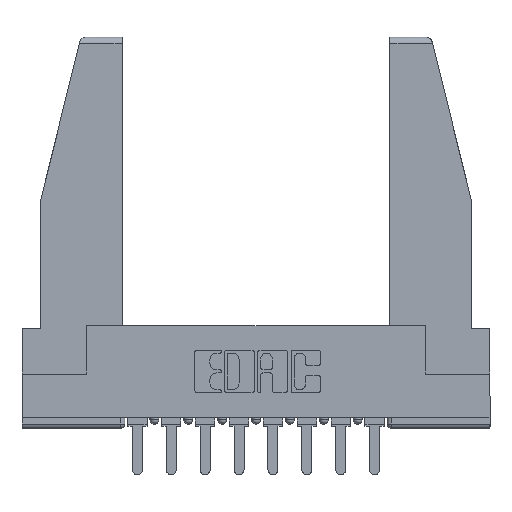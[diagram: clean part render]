
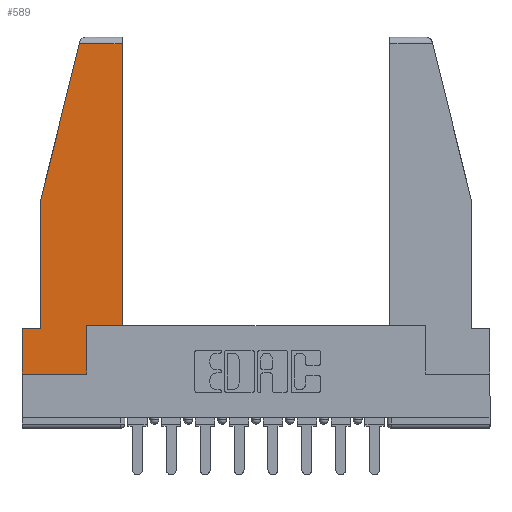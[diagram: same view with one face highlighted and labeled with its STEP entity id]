
A CAD part, top view. The second image highlights one B-rep face of the part: STEP entity #589.
In plain terms, the highlighted planar face has unit normal (0, 0, 1).
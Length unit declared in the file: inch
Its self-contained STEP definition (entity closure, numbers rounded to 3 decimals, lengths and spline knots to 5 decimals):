
#198 = CARTESIAN_POINT ( 'NONE',  ( 0.461, 0.223, 0. ) ) ;
#589 = ADVANCED_FACE ( 'NONE', ( #13682 ), #10594, .T. ) ;
#1011 = DIRECTION ( 'NONE',  ( 0., 1., 0. ) ) ;
#1154 = EDGE_CURVE ( 'NONE', #6235, #12416, #11730, .T. ) ;
#1190 = VERTEX_POINT ( 'NONE', #5610 ) ;
#1563 = LINE ( 'NONE', #4376, #9164 ) ;
#1657 = EDGE_CURVE ( 'NONE', #1190, #8794, #2591, .T. ) ;
#1777 = AXIS2_PLACEMENT_3D ( 'NONE', #8343, #13860, #11594 ) ;
#1882 = EDGE_LOOP ( 'NONE', ( #13280, #6739, #13437, #11659, #7997, #3262, #2547, #11012, #12914 ) ) ;
#1894 = EDGE_CURVE ( 'NONE', #12416, #9973, #11202, .T. ) ;
#2061 = VERTEX_POINT ( 'NONE', #4205 ) ;
#2083 = DIRECTION ( 'NONE',  ( 1., 0., 0. ) ) ;
#2334 = VECTOR ( 'NONE', #7181, 39.37008 ) ;
#2530 = LINE ( 'NONE', #5425, #10459 ) ;
#2544 = EDGE_CURVE ( 'NONE', #8794, #2061, #6162, .T. ) ;
#2547 = ORIENTED_EDGE ( 'NONE', *, *, #13365, .T. ) ;
#2591 = LINE ( 'NONE', #7949, #6899 ) ;
#3027 = LINE ( 'NONE', #4429, #4070 ) ;
#3166 = CARTESIAN_POINT ( 'NONE',  ( 0., 0.21, 0. ) ) ;
#3262 = ORIENTED_EDGE ( 'NONE', *, *, #2544, .T. ) ;
#4070 = VECTOR ( 'NONE', #1011, 39.37008 ) ;
#4136 = VECTOR ( 'NONE', #13581, 39.37008 ) ;
#4205 = CARTESIAN_POINT ( 'NONE',  ( 0., 0., 0. ) ) ;
#4376 = CARTESIAN_POINT ( 'NONE',  ( 0.297, 0.223, 0. ) ) ;
#4429 = CARTESIAN_POINT ( 'NONE',  ( 0.297, 0., 0. ) ) ;
#4791 = VECTOR ( 'NONE', #9503, 39.37008 ) ;
#4915 = LINE ( 'NONE', #12209, #12314 ) ;
#5010 = VECTOR ( 'NONE', #5769, 39.37008 ) ;
#5425 = CARTESIAN_POINT ( 'NONE',  ( 0.271, 1.55, 0. ) ) ;
#5610 = CARTESIAN_POINT ( 'NONE',  ( 0.086, 0.21, 0. ) ) ;
#5612 = CARTESIAN_POINT ( 'NONE',  ( 0.297, 0.223, 0. ) ) ;
#5769 = DIRECTION ( 'NONE',  ( 0., 1., 0. ) ) ;
#6002 = VERTEX_POINT ( 'NONE', #7423 ) ;
#6162 = LINE ( 'NONE', #8306, #4791 ) ;
#6235 = VERTEX_POINT ( 'NONE', #198 ) ;
#6728 = CARTESIAN_POINT ( 'NONE',  ( 0.461, 0.223, 0. ) ) ;
#6739 = ORIENTED_EDGE ( 'NONE', *, *, #1894, .T. ) ;
#6899 = VECTOR ( 'NONE', #13050, 39.37008 ) ;
#7181 = DIRECTION ( 'NONE',  ( 0., -1., 0. ) ) ;
#7215 = CARTESIAN_POINT ( 'NONE',  ( 0.2636, 1.52, 0. ) ) ;
#7249 = EDGE_CURVE ( 'NONE', #11210, #6235, #1563, .T. ) ;
#7423 = CARTESIAN_POINT ( 'NONE',  ( 0.086, 0.8, 0. ) ) ;
#7583 = VERTEX_POINT ( 'NONE', #13689 ) ;
#7949 = CARTESIAN_POINT ( 'NONE',  ( 0., 0.21, 0. ) ) ;
#7997 = ORIENTED_EDGE ( 'NONE', *, *, #1657, .T. ) ;
#8201 = LINE ( 'NONE', #12606, #2334 ) ;
#8306 = CARTESIAN_POINT ( 'NONE',  ( 0., 0.21, 0. ) ) ;
#8343 = CARTESIAN_POINT ( 'NONE',  ( 0., 0., 0. ) ) ;
#8708 = EDGE_CURVE ( 'NONE', #6002, #1190, #8201, .T. ) ;
#8755 = EDGE_CURVE ( 'NONE', #7583, #11210, #3027, .T. ) ;
#8767 = DIRECTION ( 'NONE',  ( 1., 0., 0. ) ) ;
#8794 = VERTEX_POINT ( 'NONE', #3166 ) ;
#9164 = VECTOR ( 'NONE', #2083, 39.37008 ) ;
#9195 = CARTESIAN_POINT ( 'NONE',  ( 0., 1.52, 0. ) ) ;
#9503 = DIRECTION ( 'NONE',  ( 0., -1., 0. ) ) ;
#9973 = VERTEX_POINT ( 'NONE', #7215 ) ;
#10135 = CARTESIAN_POINT ( 'NONE',  ( 0.461, 1.52, 0. ) ) ;
#10459 = VECTOR ( 'NONE', #10691, 39.37008 ) ;
#10594 = PLANE ( 'NONE',  #1777 ) ;
#10691 = DIRECTION ( 'NONE',  ( -0.239, -0.971, 0. ) ) ;
#11012 = ORIENTED_EDGE ( 'NONE', *, *, #8755, .T. ) ;
#11202 = LINE ( 'NONE', #9195, #4136 ) ;
#11210 = VERTEX_POINT ( 'NONE', #5612 ) ;
#11594 = DIRECTION ( 'NONE',  ( 1., 0., 0. ) ) ;
#11659 = ORIENTED_EDGE ( 'NONE', *, *, #8708, .T. ) ;
#11730 = LINE ( 'NONE', #6728, #5010 ) ;
#12209 = CARTESIAN_POINT ( 'NONE',  ( 0., 0., 0. ) ) ;
#12314 = VECTOR ( 'NONE', #8767, 39.37008 ) ;
#12416 = VERTEX_POINT ( 'NONE', #10135 ) ;
#12606 = CARTESIAN_POINT ( 'NONE',  ( 0.086, 0.8, 0. ) ) ;
#12723 = EDGE_CURVE ( 'NONE', #9973, #6002, #2530, .T. ) ;
#12914 = ORIENTED_EDGE ( 'NONE', *, *, #7249, .T. ) ;
#13050 = DIRECTION ( 'NONE',  ( -1., 0., 0. ) ) ;
#13280 = ORIENTED_EDGE ( 'NONE', *, *, #1154, .T. ) ;
#13365 = EDGE_CURVE ( 'NONE', #2061, #7583, #4915, .T. ) ;
#13437 = ORIENTED_EDGE ( 'NONE', *, *, #12723, .T. ) ;
#13581 = DIRECTION ( 'NONE',  ( -1., 0., 0. ) ) ;
#13682 = FACE_OUTER_BOUND ( 'NONE', #1882, .T. ) ;
#13689 = CARTESIAN_POINT ( 'NONE',  ( 0.297, 0., 0. ) ) ;
#13860 = DIRECTION ( 'NONE',  ( 0., 0., 1. ) ) ;
